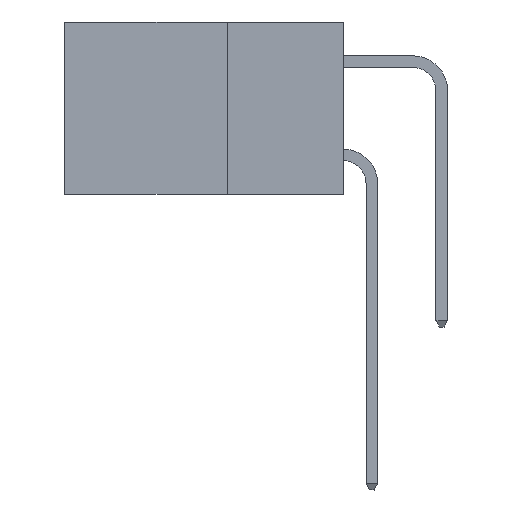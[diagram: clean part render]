
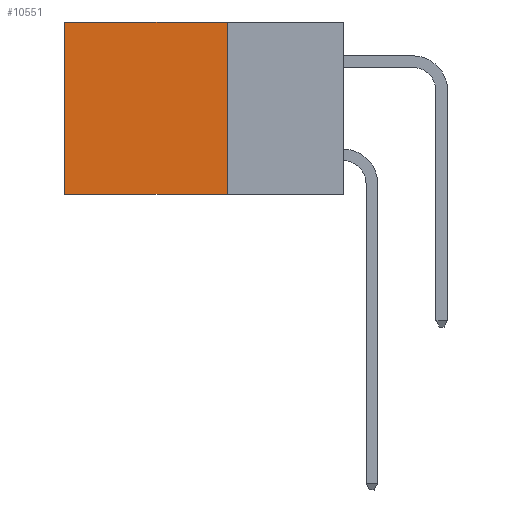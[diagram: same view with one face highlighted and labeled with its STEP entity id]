
A CAD part, left-side view. The second image highlights one B-rep face of the part: STEP entity #10551.
In plain terms, the highlighted planar face has unit normal (-1, 0, 0).
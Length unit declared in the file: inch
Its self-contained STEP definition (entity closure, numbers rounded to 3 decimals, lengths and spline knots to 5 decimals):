
#383 = LINE ( 'NONE', #13129, #9340 ) ;
#933 = FACE_OUTER_BOUND ( 'NONE', #4284, .T. ) ;
#1221 = LINE ( 'NONE', #2946, #10128 ) ;
#2309 = ORIENTED_EDGE ( 'NONE', *, *, #12785, .T. ) ;
#2946 = CARTESIAN_POINT ( 'NONE',  ( 0.298, 0.25, 0. ) ) ;
#4109 = DIRECTION ( 'NONE',  ( 1., 0., 0. ) ) ;
#4189 = DIRECTION ( 'NONE',  ( 0., 0., -1. ) ) ;
#4284 = EDGE_LOOP ( 'NONE', ( #11688, #6384, #13156, #2309 ) ) ;
#4366 = CARTESIAN_POINT ( 'NONE',  ( 0.298, 0.6, -0.37 ) ) ;
#4556 = VERTEX_POINT ( 'NONE', #10540 ) ;
#4689 = VECTOR ( 'NONE', #6693, 39.37008 ) ;
#5580 = CARTESIAN_POINT ( 'NONE',  ( 0.298, 0.25, 0. ) ) ;
#6384 = ORIENTED_EDGE ( 'NONE', *, *, #7177, .F. ) ;
#6693 = DIRECTION ( 'NONE',  ( 0., 1., 0. ) ) ;
#6766 = LINE ( 'NONE', #10655, #9762 ) ;
#6849 = VERTEX_POINT ( 'NONE', #10968 ) ;
#7177 = EDGE_CURVE ( 'NONE', #6849, #7480, #6766, .T. ) ;
#7480 = VERTEX_POINT ( 'NONE', #4366 ) ;
#8633 = CARTESIAN_POINT ( 'NONE',  ( 0.298, 0.25, 0. ) ) ;
#9340 = VECTOR ( 'NONE', #14242, 39.37008 ) ;
#9762 = VECTOR ( 'NONE', #11943, 39.37008 ) ;
#9889 = EDGE_CURVE ( 'NONE', #11661, #7480, #383, .T. ) ;
#10128 = VECTOR ( 'NONE', #4189, 39.37008 ) ;
#10540 = CARTESIAN_POINT ( 'NONE',  ( 0.298, 0.25, 0. ) ) ;
#10551 = ADVANCED_FACE ( 'NONE', ( #933 ), #10940, .F. ) ;
#10655 = CARTESIAN_POINT ( 'NONE',  ( 0.298, 0.25, -0.37 ) ) ;
#10707 = LINE ( 'NONE', #5580, #4689 ) ;
#10940 = PLANE ( 'NONE',  #11941 ) ;
#10968 = CARTESIAN_POINT ( 'NONE',  ( 0.298, 0.25, -0.37 ) ) ;
#11661 = VERTEX_POINT ( 'NONE', #13595 ) ;
#11688 = ORIENTED_EDGE ( 'NONE', *, *, #9889, .T. ) ;
#11941 = AXIS2_PLACEMENT_3D ( 'NONE', #8633, #4109, #12111 ) ;
#11943 = DIRECTION ( 'NONE',  ( 0., 1., 0. ) ) ;
#12111 = DIRECTION ( 'NONE',  ( 0., 0., -1. ) ) ;
#12785 = EDGE_CURVE ( 'NONE', #4556, #11661, #10707, .T. ) ;
#13129 = CARTESIAN_POINT ( 'NONE',  ( 0.298, 0.6, 0. ) ) ;
#13156 = ORIENTED_EDGE ( 'NONE', *, *, #13898, .F. ) ;
#13595 = CARTESIAN_POINT ( 'NONE',  ( 0.298, 0.6, 0. ) ) ;
#13898 = EDGE_CURVE ( 'NONE', #4556, #6849, #1221, .T. ) ;
#14242 = DIRECTION ( 'NONE',  ( 0., 0., -1. ) ) ;
